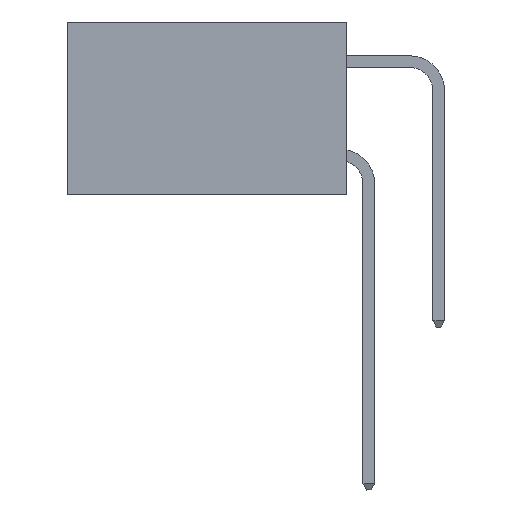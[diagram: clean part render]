
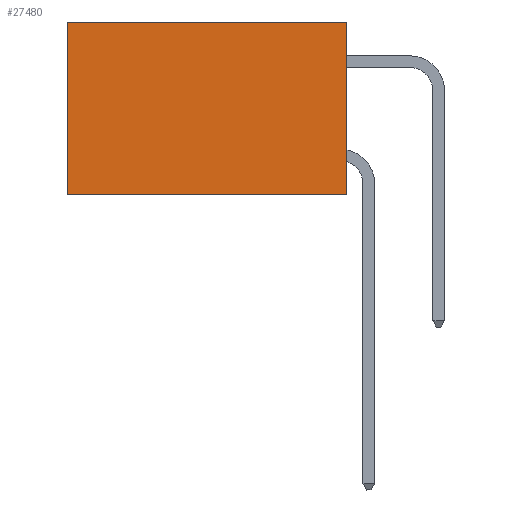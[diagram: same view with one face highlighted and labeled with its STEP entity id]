
A CAD part, left-side view. The second image highlights one B-rep face of the part: STEP entity #27480.
In plain terms, the highlighted planar face has unit normal (-1, 0, 0).
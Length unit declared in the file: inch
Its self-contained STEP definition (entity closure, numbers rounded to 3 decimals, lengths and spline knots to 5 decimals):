
#300 = CARTESIAN_POINT ( 'NONE',  ( 0.2875, 0.6, 0. ) ) ;
#562 = ORIENTED_EDGE ( 'NONE', *, *, #19212, .T. ) ;
#4163 = EDGE_CURVE ( 'NONE', #19019, #16070, #18423, .T. ) ;
#4373 = CARTESIAN_POINT ( 'NONE',  ( 0.2875, 0., 0. ) ) ;
#5289 = VECTOR ( 'NONE', #18583, 39.37008 ) ;
#5861 = CARTESIAN_POINT ( 'NONE',  ( 0.2875, 0.6, -0.37 ) ) ;
#5901 = CARTESIAN_POINT ( 'NONE',  ( 0.2875, 0., 0. ) ) ;
#5968 = CARTESIAN_POINT ( 'NONE',  ( 0.2875, 0., -0.37 ) ) ;
#6331 = AXIS2_PLACEMENT_3D ( 'NONE', #27329, #29445, #10454 ) ;
#8665 = EDGE_CURVE ( 'NONE', #13677, #9114, #23140, .T. ) ;
#9114 = VERTEX_POINT ( 'NONE', #5968 ) ;
#10454 = DIRECTION ( 'NONE',  ( 0., 0., -1. ) ) ;
#13239 = CARTESIAN_POINT ( 'NONE',  ( 0.2875, 0., -0.37 ) ) ;
#13555 = DIRECTION ( 'NONE',  ( 0., 0., -1. ) ) ;
#13677 = VERTEX_POINT ( 'NONE', #29341 ) ;
#14285 = VECTOR ( 'NONE', #17297, 39.37008 ) ;
#14306 = ORIENTED_EDGE ( 'NONE', *, *, #8665, .F. ) ;
#14568 = EDGE_CURVE ( 'NONE', #9114, #16070, #16528, .T. ) ;
#16070 = VERTEX_POINT ( 'NONE', #5861 ) ;
#16528 = LINE ( 'NONE', #13239, #5289 ) ;
#17297 = DIRECTION ( 'NONE',  ( 0., 0., -1. ) ) ;
#17462 = PLANE ( 'NONE',  #6331 ) ;
#17826 = EDGE_LOOP ( 'NONE', ( #22113, #28941, #14306, #562 ) ) ;
#18016 = CARTESIAN_POINT ( 'NONE',  ( 0.2875, 0.6, 0. ) ) ;
#18423 = LINE ( 'NONE', #300, #14285 ) ;
#18583 = DIRECTION ( 'NONE',  ( 0., 1., 0. ) ) ;
#19019 = VERTEX_POINT ( 'NONE', #18016 ) ;
#19212 = EDGE_CURVE ( 'NONE', #13677, #19019, #27867, .T. ) ;
#19775 = VECTOR ( 'NONE', #13555, 39.37008 ) ;
#20342 = VECTOR ( 'NONE', #23753, 39.37008 ) ;
#22113 = ORIENTED_EDGE ( 'NONE', *, *, #4163, .T. ) ;
#23140 = LINE ( 'NONE', #5901, #19775 ) ;
#23753 = DIRECTION ( 'NONE',  ( 0., 1., 0. ) ) ;
#27329 = CARTESIAN_POINT ( 'NONE',  ( 0.2875, 0., 0. ) ) ;
#27480 = ADVANCED_FACE ( 'NONE', ( #30115 ), #17462, .F. ) ;
#27867 = LINE ( 'NONE', #4373, #20342 ) ;
#28941 = ORIENTED_EDGE ( 'NONE', *, *, #14568, .F. ) ;
#29341 = CARTESIAN_POINT ( 'NONE',  ( 0.2875, 0., 0. ) ) ;
#29445 = DIRECTION ( 'NONE',  ( 1., 0., 0. ) ) ;
#30115 = FACE_OUTER_BOUND ( 'NONE', #17826, .T. ) ;
